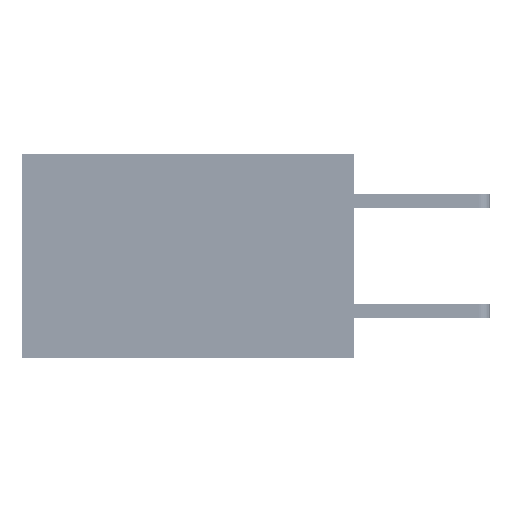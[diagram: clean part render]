
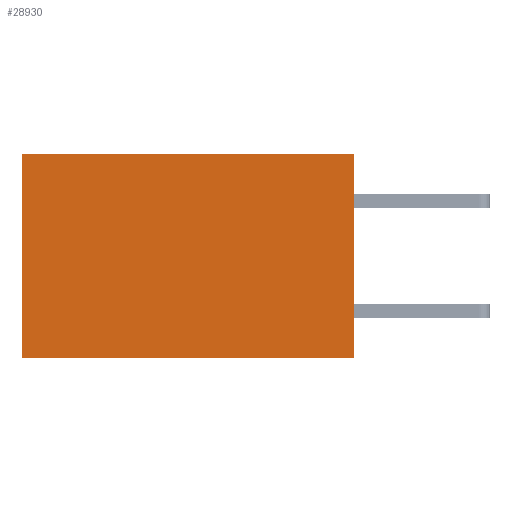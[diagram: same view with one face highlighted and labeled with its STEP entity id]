
A CAD part, left-side view. The second image highlights one B-rep face of the part: STEP entity #28930.
In plain terms, the highlighted planar face has unit normal (-1, 0, 0).
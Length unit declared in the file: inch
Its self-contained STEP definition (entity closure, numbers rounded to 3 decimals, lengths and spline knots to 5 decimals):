
#178 = EDGE_CURVE ( 'NONE', #853, #25246, #10046, .T. ) ;
#853 = VERTEX_POINT ( 'NONE', #7278 ) ;
#1009 = PLANE ( 'NONE',  #16852 ) ;
#1294 = EDGE_CURVE ( 'NONE', #21855, #8991, #24599, .T. ) ;
#2930 = DIRECTION ( 'NONE',  ( 0., 0., -1. ) ) ;
#4272 = DIRECTION ( 'NONE',  ( 0., 0., -1. ) ) ;
#6489 = CARTESIAN_POINT ( 'NONE',  ( 0.2875, 0.6, 0. ) ) ;
#6664 = FACE_OUTER_BOUND ( 'NONE', #28630, .T. ) ;
#7278 = CARTESIAN_POINT ( 'NONE',  ( 0.2875, 0., -0.37 ) ) ;
#8991 = VERTEX_POINT ( 'NONE', #6489 ) ;
#10046 = LINE ( 'NONE', #38006, #29159 ) ;
#10734 = EDGE_CURVE ( 'NONE', #21855, #853, #11260, .T. ) ;
#11260 = LINE ( 'NONE', #23545, #21872 ) ;
#11287 = CARTESIAN_POINT ( 'NONE',  ( 0.2875, 0., 0. ) ) ;
#14199 = DIRECTION ( 'NONE',  ( 0., 0., -1. ) ) ;
#16852 = AXIS2_PLACEMENT_3D ( 'NONE', #26775, #23521, #14199 ) ;
#18959 = LINE ( 'NONE', #22330, #23048 ) ;
#20899 = ORIENTED_EDGE ( 'NONE', *, *, #178, .F. ) ;
#21855 = VERTEX_POINT ( 'NONE', #11287 ) ;
#21872 = VECTOR ( 'NONE', #4272, 39.37008 ) ;
#22330 = CARTESIAN_POINT ( 'NONE',  ( 0.2875, 0.6, 0. ) ) ;
#23048 = VECTOR ( 'NONE', #2930, 39.37008 ) ;
#23521 = DIRECTION ( 'NONE',  ( 1., 0., 0. ) ) ;
#23545 = CARTESIAN_POINT ( 'NONE',  ( 0.2875, 0., 0. ) ) ;
#24599 = LINE ( 'NONE', #26235, #30569 ) ;
#25246 = VERTEX_POINT ( 'NONE', #35828 ) ;
#26235 = CARTESIAN_POINT ( 'NONE',  ( 0.2875, 0., 0. ) ) ;
#26775 = CARTESIAN_POINT ( 'NONE',  ( 0.2875, 0., 0. ) ) ;
#27226 = ORIENTED_EDGE ( 'NONE', *, *, #1294, .T. ) ;
#28630 = EDGE_LOOP ( 'NONE', ( #36638, #20899, #31589, #27226 ) ) ;
#28930 = ADVANCED_FACE ( 'NONE', ( #6664 ), #1009, .F. ) ;
#29159 = VECTOR ( 'NONE', #41396, 39.37008 ) ;
#30569 = VECTOR ( 'NONE', #39170, 39.37008 ) ;
#31589 = ORIENTED_EDGE ( 'NONE', *, *, #10734, .F. ) ;
#31832 = EDGE_CURVE ( 'NONE', #8991, #25246, #18959, .T. ) ;
#35828 = CARTESIAN_POINT ( 'NONE',  ( 0.2875, 0.6, -0.37 ) ) ;
#36638 = ORIENTED_EDGE ( 'NONE', *, *, #31832, .T. ) ;
#38006 = CARTESIAN_POINT ( 'NONE',  ( 0.2875, 0., -0.37 ) ) ;
#39170 = DIRECTION ( 'NONE',  ( 0., 1., 0. ) ) ;
#41396 = DIRECTION ( 'NONE',  ( 0., 1., 0. ) ) ;
